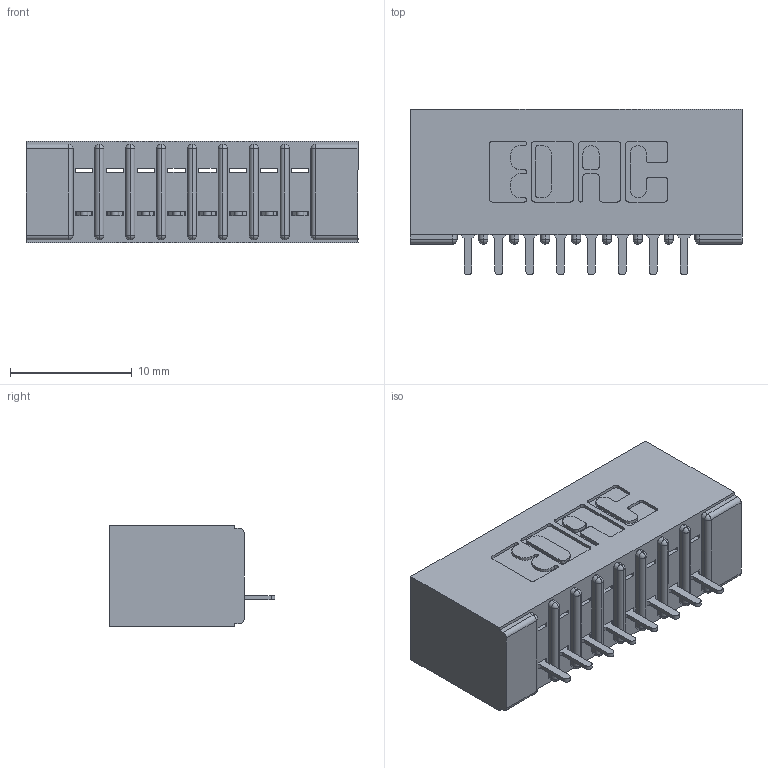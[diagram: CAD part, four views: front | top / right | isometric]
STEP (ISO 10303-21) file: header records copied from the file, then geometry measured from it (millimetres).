
FILE_DESCRIPTION (( 'STEP AP203' ), '1' );
FILE_NAME ('391-008-524-101.STEP', '2018-08-08T15:38:22', ( '' ), ( '' ), 'SwSTEP 2.0', 'SolidWorks 2016', '' );
FILE_SCHEMA (( 'CONFIG_CONTROL_DESIGN' ));
Length unit declared in the file: inch
Products named in the file (3): 341 Part_No Mounting Lugs; 341-292-001_341-292-124; 391-008-524-101
Assembly tree (9 placements, depth 2):
  391-008-524-101
    341 Part_No Mounting Lugs
    341-292-001_341-292-124  x8
Bounding box: 27.3 x 13.64 x 8.38 mm (x, y, z)
Volume: 1663.5 mm3; surface area: 2883 mm2
Topology: 9 solids, 9 shells, 764 faces, 2188 edges, 1406 vertices
Faces by surface type: plane 472, cylinder 260, sphere 18, torus 14
Entity records: 13677 total; most frequent: CARTESIAN_POINT 2308, ORIENTED_EDGE 2296, DIRECTION 2254, EDGE_CURVE 1148, VECTOR 894, LINE 894, VERTEX_POINT 734, AXIS2_PLACEMENT_3D 680
